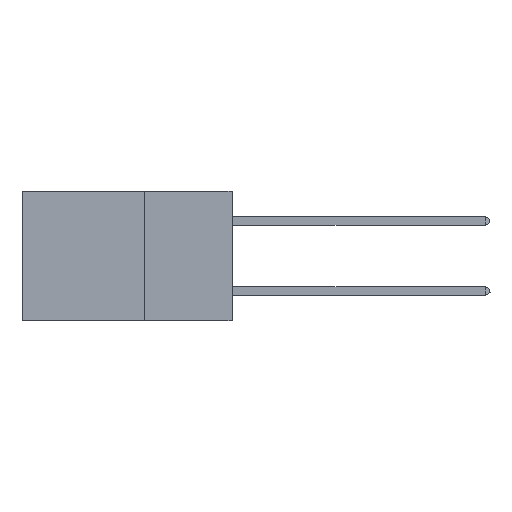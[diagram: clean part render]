
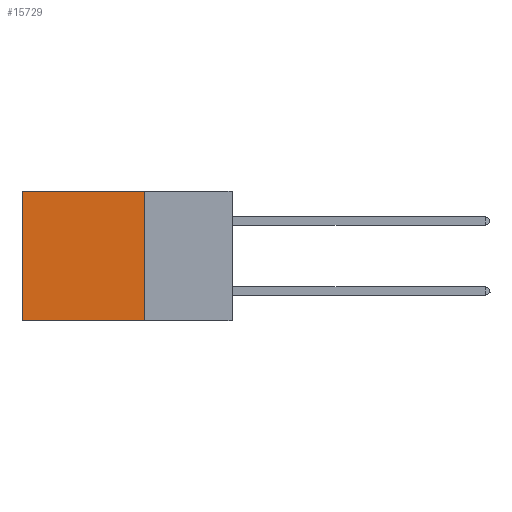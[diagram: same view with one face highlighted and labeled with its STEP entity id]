
A CAD part, left-side view. The second image highlights one B-rep face of the part: STEP entity #15729.
In plain terms, the highlighted planar face has unit normal (-1, 0, 0).
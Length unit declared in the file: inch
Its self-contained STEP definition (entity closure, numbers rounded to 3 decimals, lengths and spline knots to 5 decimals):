
#33 = CARTESIAN_POINT ( 'NONE',  ( 0.2875, 0.6, -0.37 ) ) ;
#1307 = DIRECTION ( 'NONE',  ( 0., 0., -1. ) ) ;
#1491 = ORIENTED_EDGE ( 'NONE', *, *, #21206, .T. ) ;
#3015 = VERTEX_POINT ( 'NONE', #33 ) ;
#7460 = ORIENTED_EDGE ( 'NONE', *, *, #18302, .F. ) ;
#8360 = LINE ( 'NONE', #22600, #15898 ) ;
#8891 = DIRECTION ( 'NONE',  ( 0., 1., 0. ) ) ;
#9815 = DIRECTION ( 'NONE',  ( 0., 0., -1. ) ) ;
#10064 = CARTESIAN_POINT ( 'NONE',  ( 0.2875, 0.25, -0.37 ) ) ;
#11630 = VECTOR ( 'NONE', #1307, 39.37008 ) ;
#11907 = EDGE_CURVE ( 'NONE', #14407, #3015, #12315, .T. ) ;
#11948 = CARTESIAN_POINT ( 'NONE',  ( 0.2875, 0.25, 0. ) ) ;
#12315 = LINE ( 'NONE', #26581, #11630 ) ;
#12603 = VERTEX_POINT ( 'NONE', #10064 ) ;
#12686 = CARTESIAN_POINT ( 'NONE',  ( 0.2875, 0.6, 0. ) ) ;
#13042 = FACE_OUTER_BOUND ( 'NONE', #16909, .T. ) ;
#13672 = VERTEX_POINT ( 'NONE', #17798 ) ;
#14407 = VERTEX_POINT ( 'NONE', #12686 ) ;
#15018 = CARTESIAN_POINT ( 'NONE',  ( 0.2875, 0.25, -0.37 ) ) ;
#15729 = ADVANCED_FACE ( 'NONE', ( #13042 ), #24443, .F. ) ;
#15898 = VECTOR ( 'NONE', #18429, 39.37008 ) ;
#16453 = VECTOR ( 'NONE', #8891, 39.37008 ) ;
#16909 = EDGE_LOOP ( 'NONE', ( #26288, #17055, #7460, #1491 ) ) ;
#17055 = ORIENTED_EDGE ( 'NONE', *, *, #17192, .F. ) ;
#17192 = EDGE_CURVE ( 'NONE', #12603, #3015, #24649, .T. ) ;
#17798 = CARTESIAN_POINT ( 'NONE',  ( 0.2875, 0.25, 0. ) ) ;
#18302 = EDGE_CURVE ( 'NONE', #13672, #12603, #26535, .T. ) ;
#18334 = DIRECTION ( 'NONE',  ( 1., 0., 0. ) ) ;
#18429 = DIRECTION ( 'NONE',  ( 0., 1., 0. ) ) ;
#18451 = AXIS2_PLACEMENT_3D ( 'NONE', #11948, #18334, #9815 ) ;
#18552 = DIRECTION ( 'NONE',  ( 0., 0., -1. ) ) ;
#18729 = CARTESIAN_POINT ( 'NONE',  ( 0.2875, 0.25, 0. ) ) ;
#20990 = VECTOR ( 'NONE', #18552, 39.37008 ) ;
#21206 = EDGE_CURVE ( 'NONE', #13672, #14407, #8360, .T. ) ;
#22600 = CARTESIAN_POINT ( 'NONE',  ( 0.2875, 0.25, 0. ) ) ;
#24443 = PLANE ( 'NONE',  #18451 ) ;
#24649 = LINE ( 'NONE', #15018, #16453 ) ;
#26288 = ORIENTED_EDGE ( 'NONE', *, *, #11907, .T. ) ;
#26535 = LINE ( 'NONE', #18729, #20990 ) ;
#26581 = CARTESIAN_POINT ( 'NONE',  ( 0.2875, 0.6, 0. ) ) ;
